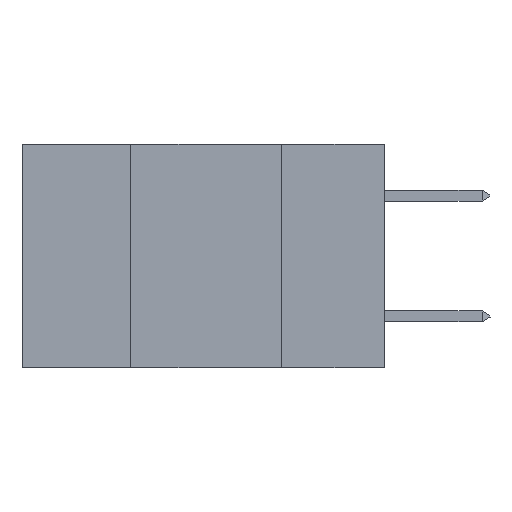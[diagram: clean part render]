
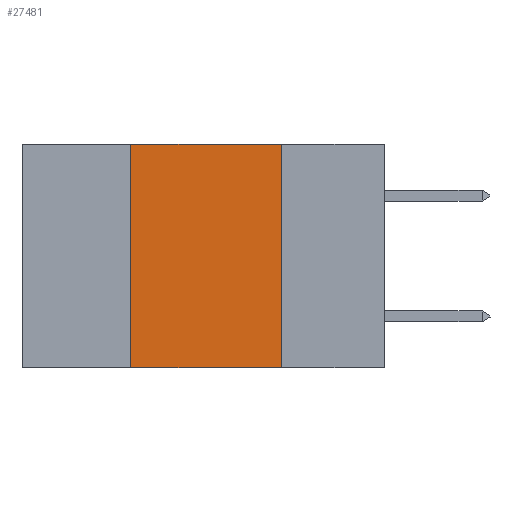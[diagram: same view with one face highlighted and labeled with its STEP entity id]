
A CAD part, left-side view. The second image highlights one B-rep face of the part: STEP entity #27481.
In plain terms, the highlighted planar face has unit normal (-1, 0, 0).
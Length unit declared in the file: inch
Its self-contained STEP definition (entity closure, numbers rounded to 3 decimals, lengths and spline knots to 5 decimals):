
#1362 = CARTESIAN_POINT ( 'NONE',  ( 0., 0.42, -0.37 ) ) ;
#1692 = EDGE_CURVE ( 'NONE', #24000, #15716, #7770, .T. ) ;
#4050 = VERTEX_POINT ( 'NONE', #14501 ) ;
#4119 = EDGE_CURVE ( 'NONE', #12731, #15716, #10457, .T. ) ;
#5187 = ORIENTED_EDGE ( 'NONE', *, *, #12160, .F. ) ;
#5655 = VECTOR ( 'NONE', #15736, 39.37008 ) ;
#5807 = LINE ( 'NONE', #28247, #25131 ) ;
#6640 = CARTESIAN_POINT ( 'NONE',  ( 0., 0.6, 0. ) ) ;
#7378 = LINE ( 'NONE', #17662, #11972 ) ;
#7747 = ORIENTED_EDGE ( 'NONE', *, *, #1692, .T. ) ;
#7770 = LINE ( 'NONE', #13484, #5655 ) ;
#8293 = CARTESIAN_POINT ( 'NONE',  ( 0., 0.17, 0. ) ) ;
#8777 = EDGE_CURVE ( 'NONE', #24000, #4050, #5807, .T. ) ;
#10457 = LINE ( 'NONE', #8293, #27739 ) ;
#11972 = VECTOR ( 'NONE', #17761, 39.37008 ) ;
#12160 = EDGE_CURVE ( 'NONE', #4050, #12731, #7378, .T. ) ;
#12731 = VERTEX_POINT ( 'NONE', #20828 ) ;
#13484 = CARTESIAN_POINT ( 'NONE',  ( 0., 0.6, -0.37 ) ) ;
#14501 = CARTESIAN_POINT ( 'NONE',  ( 0., 0.42, 0. ) ) ;
#15470 = DIRECTION ( 'NONE',  ( 1., 0., 0. ) ) ;
#15716 = VERTEX_POINT ( 'NONE', #23588 ) ;
#15736 = DIRECTION ( 'NONE',  ( 0., -1., 0. ) ) ;
#16782 = AXIS2_PLACEMENT_3D ( 'NONE', #6640, #15470, #26677 ) ;
#17118 = DIRECTION ( 'NONE',  ( 0., 0., -1. ) ) ;
#17662 = CARTESIAN_POINT ( 'NONE',  ( 0., 0.6, 0. ) ) ;
#17761 = DIRECTION ( 'NONE',  ( 0., -1., 0. ) ) ;
#18861 = FACE_OUTER_BOUND ( 'NONE', #22801, .T. ) ;
#20729 = ORIENTED_EDGE ( 'NONE', *, *, #4119, .F. ) ;
#20828 = CARTESIAN_POINT ( 'NONE',  ( 0., 0.17, 0. ) ) ;
#22801 = EDGE_LOOP ( 'NONE', ( #20729, #5187, #23728, #7747 ) ) ;
#23588 = CARTESIAN_POINT ( 'NONE',  ( 0., 0.17, -0.37 ) ) ;
#23728 = ORIENTED_EDGE ( 'NONE', *, *, #8777, .F. ) ;
#24000 = VERTEX_POINT ( 'NONE', #1362 ) ;
#25131 = VECTOR ( 'NONE', #27941, 39.37008 ) ;
#26677 = DIRECTION ( 'NONE',  ( 0., 0., -1. ) ) ;
#27033 = PLANE ( 'NONE',  #16782 ) ;
#27481 = ADVANCED_FACE ( 'NONE', ( #18861 ), #27033, .F. ) ;
#27739 = VECTOR ( 'NONE', #17118, 39.37008 ) ;
#27941 = DIRECTION ( 'NONE',  ( 0., 0., 1. ) ) ;
#28247 = CARTESIAN_POINT ( 'NONE',  ( 0., 0.42, 0. ) ) ;
